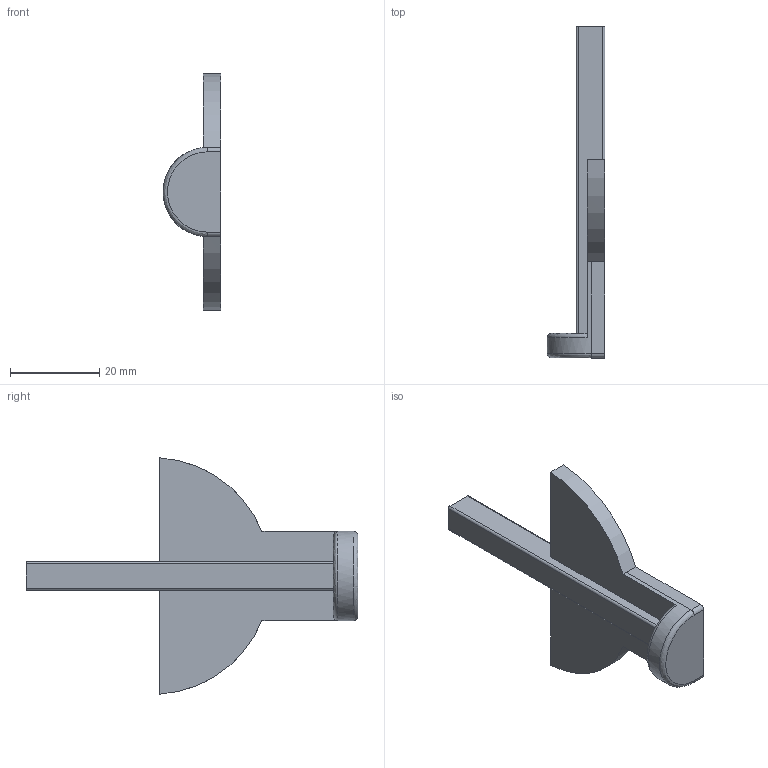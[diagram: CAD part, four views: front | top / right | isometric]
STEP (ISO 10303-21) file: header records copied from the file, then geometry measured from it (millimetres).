
FILE_DESCRIPTION (( 'STEP AP203' ), '1' );
FILE_NAME ('LOCK.STEP', '2020-09-28T01:16:03', ( '' ), ( '' ), 'SwSTEP 2.0', 'SolidWorks 2019', '' );
FILE_SCHEMA (( 'CONFIG_CONTROL_DESIGN' ));
Length unit declared in the file: millimetre
Products named in the file (1): LOCK
Bounding box: 13 x 74.51 x 53.07 mm (x, y, z)
Volume: 8192 mm3; surface area: 4971.3 mm2
Topology: 1 solids, 1 shells, 27 faces, 70 edges, 46 vertices
Faces by surface type: plane 14, cylinder 11, bspline 2
Entity records: 941 total; most frequent: CARTESIAN_POINT 200, ORIENTED_EDGE 140, DIRECTION 138, EDGE_CURVE 70, AXIS2_PLACEMENT_3D 48, VERTEX_POINT 46, LINE 42, VECTOR 42
